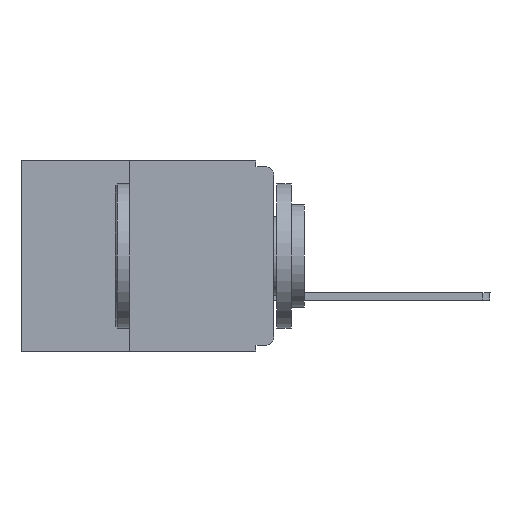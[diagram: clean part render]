
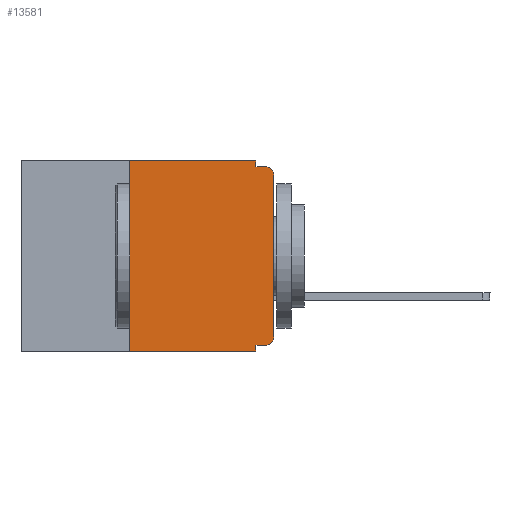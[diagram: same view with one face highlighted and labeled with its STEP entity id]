
A CAD part, left-side view. The second image highlights one B-rep face of the part: STEP entity #13581.
In plain terms, the highlighted planar face has unit normal (-1, 0, 0).
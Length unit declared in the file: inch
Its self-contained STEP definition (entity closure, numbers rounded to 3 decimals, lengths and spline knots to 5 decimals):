
#62 = EDGE_CURVE ( 'NONE', #3746, #3007, #8747, .T. ) ;
#338 = CARTESIAN_POINT ( 'NONE',  ( 0., 0.031, 0. ) ) ;
#498 = EDGE_CURVE ( 'NONE', #11826, #3746, #12652, .T. ) ;
#878 = CARTESIAN_POINT ( 'NONE',  ( 0., 0.25, -0.33 ) ) ;
#1204 = ORIENTED_EDGE ( 'NONE', *, *, #6493, .F. ) ;
#1364 = VERTEX_POINT ( 'NONE', #16474 ) ;
#1497 = EDGE_CURVE ( 'NONE', #16586, #15032, #7039, .T. ) ;
#2312 = CARTESIAN_POINT ( 'NONE',  ( 0., 0.015, -0.025 ) ) ;
#2380 = CARTESIAN_POINT ( 'NONE',  ( 0., 0., -0.305 ) ) ;
#2441 = CIRCLE ( 'NONE', #4679, 0.015 ) ;
#2975 = ORIENTED_EDGE ( 'NONE', *, *, #6743, .F. ) ;
#3007 = VERTEX_POINT ( 'NONE', #6773 ) ;
#3112 = VERTEX_POINT ( 'NONE', #9499 ) ;
#3232 = ORIENTED_EDGE ( 'NONE', *, *, #7405, .T. ) ;
#3746 = VERTEX_POINT ( 'NONE', #6877 ) ;
#3833 = CARTESIAN_POINT ( 'NONE',  ( 0., 0.437, 0. ) ) ;
#3915 = DIRECTION ( 'NONE',  ( 0., 1., 0. ) ) ;
#4570 = CARTESIAN_POINT ( 'NONE',  ( 0., 0.25, -0.33 ) ) ;
#4627 = ORIENTED_EDGE ( 'NONE', *, *, #17112, .T. ) ;
#4679 = AXIS2_PLACEMENT_3D ( 'NONE', #2312, #12401, #13860 ) ;
#4876 = VECTOR ( 'NONE', #7638, 39.37008 ) ;
#5345 = VERTEX_POINT ( 'NONE', #13856 ) ;
#5357 = DIRECTION ( 'NONE',  ( 0., 0., 1. ) ) ;
#5481 = ORIENTED_EDGE ( 'NONE', *, *, #498, .F. ) ;
#5581 = CARTESIAN_POINT ( 'NONE',  ( 0., 0.031, -0.32 ) ) ;
#5839 = VECTOR ( 'NONE', #15727, 39.37008 ) ;
#5952 = VERTEX_POINT ( 'NONE', #2380 ) ;
#6007 = AXIS2_PLACEMENT_3D ( 'NONE', #13194, #6546, #11913 ) ;
#6165 = DIRECTION ( 'NONE',  ( 0., -1., 0. ) ) ;
#6243 = ORIENTED_EDGE ( 'NONE', *, *, #8576, .T. ) ;
#6333 = CARTESIAN_POINT ( 'NONE',  ( 0., 0., -0.32 ) ) ;
#6493 = EDGE_CURVE ( 'NONE', #15032, #5345, #12947, .T. ) ;
#6546 = DIRECTION ( 'NONE',  ( 1., 0., 0. ) ) ;
#6743 = EDGE_CURVE ( 'NONE', #3007, #7971, #9005, .T. ) ;
#6773 = CARTESIAN_POINT ( 'NONE',  ( 0., 0.031, 0. ) ) ;
#6877 = CARTESIAN_POINT ( 'NONE',  ( 0., 0.25, 0. ) ) ;
#6879 = DIRECTION ( 'NONE',  ( -1., 0., 0. ) ) ;
#7039 = LINE ( 'NONE', #6333, #13663 ) ;
#7405 = EDGE_CURVE ( 'NONE', #5952, #3112, #14991, .T. ) ;
#7487 = ORIENTED_EDGE ( 'NONE', *, *, #62, .F. ) ;
#7579 = EDGE_CURVE ( 'NONE', #7971, #1364, #15392, .T. ) ;
#7638 = DIRECTION ( 'NONE',  ( 0., 0., -1. ) ) ;
#7810 = DIRECTION ( 'NONE',  ( 0., -1., 0. ) ) ;
#7971 = VERTEX_POINT ( 'NONE', #9912 ) ;
#8051 = EDGE_CURVE ( 'NONE', #16586, #5952, #14142, .T. ) ;
#8576 = EDGE_CURVE ( 'NONE', #11826, #5345, #10622, .T. ) ;
#8747 = LINE ( 'NONE', #3833, #12045 ) ;
#9005 = LINE ( 'NONE', #338, #11696 ) ;
#9499 = CARTESIAN_POINT ( 'NONE',  ( 0., 0., -0.025 ) ) ;
#9912 = CARTESIAN_POINT ( 'NONE',  ( 0., 0.031, -0.01 ) ) ;
#10622 = LINE ( 'NONE', #15281, #5839 ) ;
#11059 = CARTESIAN_POINT ( 'NONE',  ( 0., 0.015, -0.305 ) ) ;
#11212 = CARTESIAN_POINT ( 'NONE',  ( 0., 0., -0.01 ) ) ;
#11542 = EDGE_LOOP ( 'NONE', ( #3232, #4627, #14687, #2975, #7487, #5481, #6243, #1204, #14145, #14953 ) ) ;
#11696 = VECTOR ( 'NONE', #13541, 39.37008 ) ;
#11794 = PLANE ( 'NONE',  #6007 ) ;
#11826 = VERTEX_POINT ( 'NONE', #4570 ) ;
#11913 = DIRECTION ( 'NONE',  ( 0., 0., -1. ) ) ;
#12045 = VECTOR ( 'NONE', #7810, 39.37008 ) ;
#12401 = DIRECTION ( 'NONE',  ( -1., 0., 0. ) ) ;
#12652 = LINE ( 'NONE', #878, #14112 ) ;
#12947 = LINE ( 'NONE', #14023, #4876 ) ;
#13109 = VECTOR ( 'NONE', #6165, 39.37008 ) ;
#13194 = CARTESIAN_POINT ( 'NONE',  ( 0., 0.437, 0. ) ) ;
#13279 = CARTESIAN_POINT ( 'NONE',  ( 0., 0., 0. ) ) ;
#13541 = DIRECTION ( 'NONE',  ( 0., 0., -1. ) ) ;
#13581 = ADVANCED_FACE ( 'NONE', ( #17073 ), #11794, .F. ) ;
#13663 = VECTOR ( 'NONE', #3915, 39.37008 ) ;
#13856 = CARTESIAN_POINT ( 'NONE',  ( 0., 0.031, -0.33 ) ) ;
#13860 = DIRECTION ( 'NONE',  ( 0., 0., -1. ) ) ;
#14023 = CARTESIAN_POINT ( 'NONE',  ( 0., 0.031, -0.33 ) ) ;
#14112 = VECTOR ( 'NONE', #14550, 39.37008 ) ;
#14142 = CIRCLE ( 'NONE', #14473, 0.015 ) ;
#14145 = ORIENTED_EDGE ( 'NONE', *, *, #1497, .F. ) ;
#14228 = CARTESIAN_POINT ( 'NONE',  ( 0., 0.015, -0.32 ) ) ;
#14473 = AXIS2_PLACEMENT_3D ( 'NONE', #11059, #6879, #14914 ) ;
#14550 = DIRECTION ( 'NONE',  ( 0., 0., 1. ) ) ;
#14687 = ORIENTED_EDGE ( 'NONE', *, *, #7579, .F. ) ;
#14914 = DIRECTION ( 'NONE',  ( 0., 0., -1. ) ) ;
#14953 = ORIENTED_EDGE ( 'NONE', *, *, #8051, .T. ) ;
#14991 = LINE ( 'NONE', #13279, #15214 ) ;
#15032 = VERTEX_POINT ( 'NONE', #5581 ) ;
#15214 = VECTOR ( 'NONE', #5357, 39.37008 ) ;
#15281 = CARTESIAN_POINT ( 'NONE',  ( 0., 0.437, -0.33 ) ) ;
#15392 = LINE ( 'NONE', #11212, #13109 ) ;
#15727 = DIRECTION ( 'NONE',  ( 0., -1., 0. ) ) ;
#16474 = CARTESIAN_POINT ( 'NONE',  ( 0., 0.015, -0.01 ) ) ;
#16586 = VERTEX_POINT ( 'NONE', #14228 ) ;
#17073 = FACE_OUTER_BOUND ( 'NONE', #11542, .T. ) ;
#17112 = EDGE_CURVE ( 'NONE', #3112, #1364, #2441, .T. ) ;
